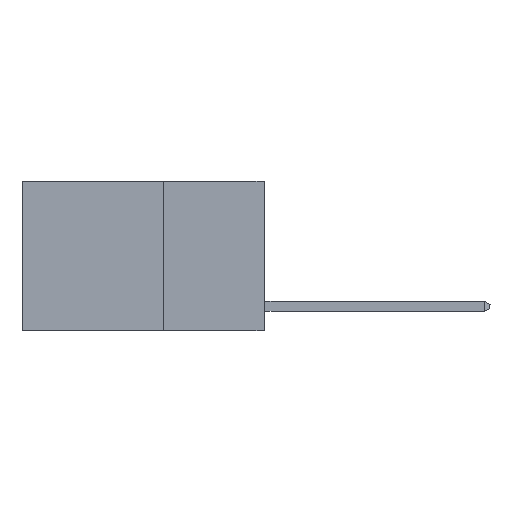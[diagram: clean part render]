
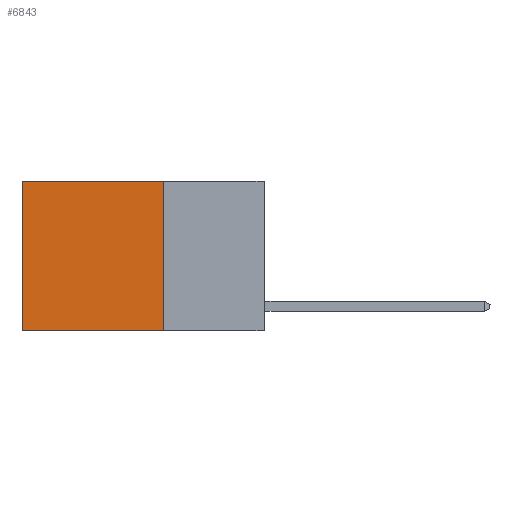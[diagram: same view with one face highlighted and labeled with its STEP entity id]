
A CAD part, left-side view. The second image highlights one B-rep face of the part: STEP entity #6843.
In plain terms, the highlighted planar face has unit normal (-1, 0, 0).
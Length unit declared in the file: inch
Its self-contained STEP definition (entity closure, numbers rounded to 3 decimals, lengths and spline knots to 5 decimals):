
#66 = VERTEX_POINT ( 'NONE', #8827 ) ;
#974 = DIRECTION ( 'NONE',  ( 0., 0., -1. ) ) ;
#1446 = ORIENTED_EDGE ( 'NONE', *, *, #17870, .T. ) ;
#1809 = EDGE_CURVE ( 'NONE', #8886, #66, #13872, .T. ) ;
#2640 = FACE_OUTER_BOUND ( 'NONE', #18111, .T. ) ;
#2735 = LINE ( 'NONE', #13860, #17245 ) ;
#4172 = VERTEX_POINT ( 'NONE', #13929 ) ;
#5979 = ORIENTED_EDGE ( 'NONE', *, *, #6692, .F. ) ;
#6358 = CARTESIAN_POINT ( 'NONE',  ( 0.2625, 0.25, 0. ) ) ;
#6692 = EDGE_CURVE ( 'NONE', #4172, #8886, #7296, .T. ) ;
#6843 = ADVANCED_FACE ( 'NONE', ( #2640 ), #12318, .F. ) ;
#7296 = LINE ( 'NONE', #16850, #11384 ) ;
#8827 = CARTESIAN_POINT ( 'NONE',  ( 0.2625, 0.6, -0.37 ) ) ;
#8886 = VERTEX_POINT ( 'NONE', #18775 ) ;
#9137 = ORIENTED_EDGE ( 'NONE', *, *, #22393, .T. ) ;
#9441 = ORIENTED_EDGE ( 'NONE', *, *, #1809, .F. ) ;
#9769 = VECTOR ( 'NONE', #18456, 39.37008 ) ;
#10222 = DIRECTION ( 'NONE',  ( 0., 0., -1. ) ) ;
#10913 = DIRECTION ( 'NONE',  ( 0., 1., 0. ) ) ;
#11384 = VECTOR ( 'NONE', #974, 39.37008 ) ;
#12318 = PLANE ( 'NONE',  #21067 ) ;
#12807 = LINE ( 'NONE', #6358, #9769 ) ;
#13860 = CARTESIAN_POINT ( 'NONE',  ( 0.2625, 0.6, 0. ) ) ;
#13872 = LINE ( 'NONE', #14742, #22042 ) ;
#13929 = CARTESIAN_POINT ( 'NONE',  ( 0.2625, 0.25, 0. ) ) ;
#14742 = CARTESIAN_POINT ( 'NONE',  ( 0.2625, 0.25, -0.37 ) ) ;
#15797 = DIRECTION ( 'NONE',  ( 0., 0., -1. ) ) ;
#16850 = CARTESIAN_POINT ( 'NONE',  ( 0.2625, 0.25, 0. ) ) ;
#16927 = VERTEX_POINT ( 'NONE', #19256 ) ;
#17245 = VECTOR ( 'NONE', #10222, 39.37008 ) ;
#17870 = EDGE_CURVE ( 'NONE', #16927, #66, #2735, .T. ) ;
#18111 = EDGE_LOOP ( 'NONE', ( #1446, #9441, #5979, #9137 ) ) ;
#18456 = DIRECTION ( 'NONE',  ( 0., 1., 0. ) ) ;
#18775 = CARTESIAN_POINT ( 'NONE',  ( 0.2625, 0.25, -0.37 ) ) ;
#19256 = CARTESIAN_POINT ( 'NONE',  ( 0.2625, 0.6, 0. ) ) ;
#21067 = AXIS2_PLACEMENT_3D ( 'NONE', #21100, #22638, #15797 ) ;
#21100 = CARTESIAN_POINT ( 'NONE',  ( 0.2625, 0.25, 0. ) ) ;
#22042 = VECTOR ( 'NONE', #10913, 39.37008 ) ;
#22393 = EDGE_CURVE ( 'NONE', #4172, #16927, #12807, .T. ) ;
#22638 = DIRECTION ( 'NONE',  ( 1., 0., 0. ) ) ;
